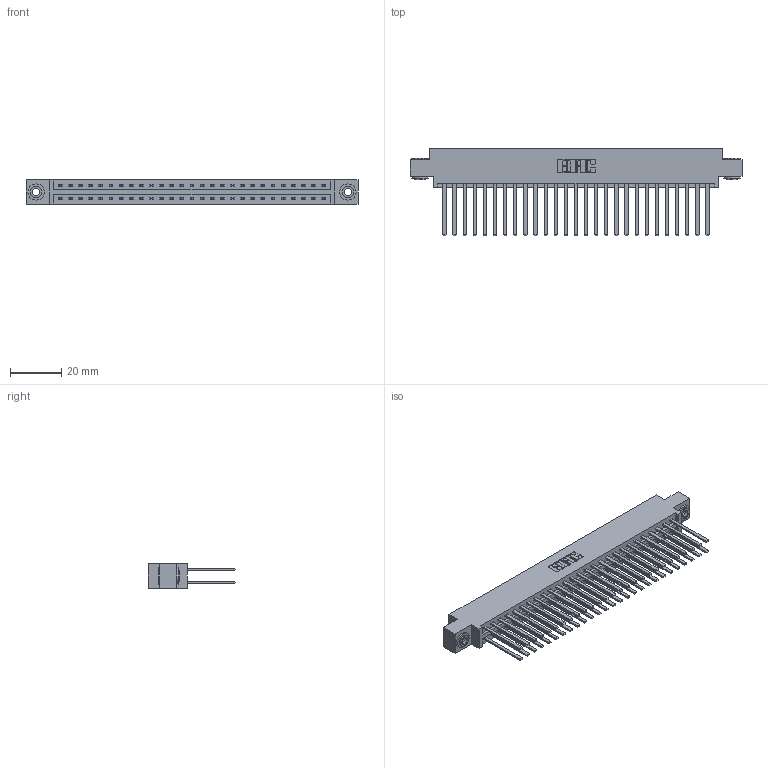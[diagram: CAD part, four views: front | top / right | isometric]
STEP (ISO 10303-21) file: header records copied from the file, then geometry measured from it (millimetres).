
FILE_DESCRIPTION (( 'STEP AP203' ), '1' );
FILE_NAME ('337-054-544-803.STEP', '2019-10-11T19:08:34', ( '' ), ( '' ), 'SwSTEP 2.0', 'SolidWorks 2016', '' );
FILE_SCHEMA (( 'CONFIG_CONTROL_DESIGN' ));
Length unit declared in the file: inch
Products named in the file (4): 345-292-001_345-293-144; 337-054-544-803; 345-250-002_345-250-002-102; 337 Part_0.170 Offset - 0.156 Dia-TH
Assembly tree (57 placements, depth 2):
  337-054-544-803
    337 Part_0.170 Offset - 0.156 Dia-TH
    345-292-001_345-293-144  x54
    345-250-002_345-250-002-102  x2
Bounding box: 130 x 34.3 x 9.4 mm (x, y, z)
Volume: 14159.3 mm3; surface area: 18666.5 mm2
Topology: 57 solids, 57 shells, 2748 faces, 8121 edges, 5338 vertices
Faces by surface type: plane 1920, cylinder 820, cone 8
Entity records: 23472 total; most frequent: CARTESIAN_POINT 3941, ORIENTED_EDGE 3870, DIRECTION 3409, EDGE_CURVE 1935, VECTOR 1787, LINE 1787, VERTEX_POINT 1286, AXIS2_PLACEMENT_3D 811
